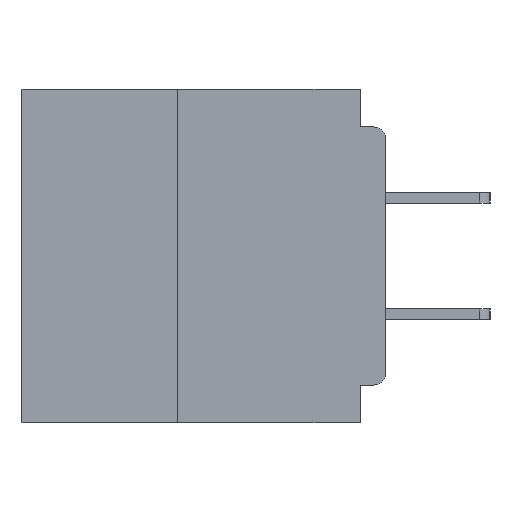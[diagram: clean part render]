
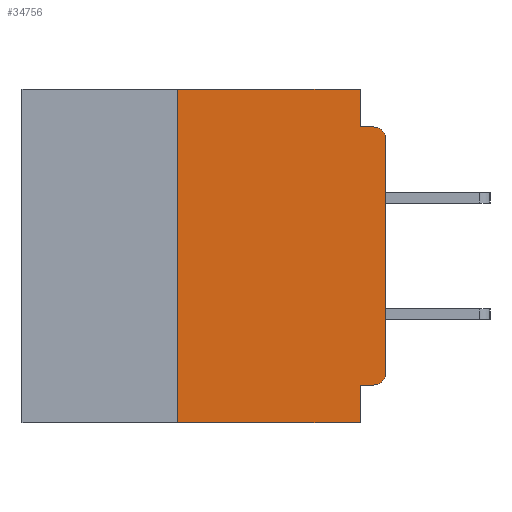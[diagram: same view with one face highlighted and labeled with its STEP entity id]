
A CAD part, left-side view. The second image highlights one B-rep face of the part: STEP entity #34756.
In plain terms, the highlighted planar face has unit normal (-1, 0, 0).
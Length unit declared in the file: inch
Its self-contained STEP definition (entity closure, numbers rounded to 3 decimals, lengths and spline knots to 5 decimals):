
#639 = LINE ( 'NONE', #32793, #15020 ) ;
#721 = ORIENTED_EDGE ( 'NONE', *, *, #3577, .T. ) ;
#1057 = ORIENTED_EDGE ( 'NONE', *, *, #13019, .F. ) ;
#1140 = ORIENTED_EDGE ( 'NONE', *, *, #12004, .T. ) ;
#1785 = VECTOR ( 'NONE', #26049, 39.37008 ) ;
#1883 = DIRECTION ( 'NONE',  ( 0., 0., -1. ) ) ;
#1894 = VERTEX_POINT ( 'NONE', #34865 ) ;
#2297 = DIRECTION ( 'NONE',  ( 0., 0., -1. ) ) ;
#2984 = CARTESIAN_POINT ( 'NONE',  ( 0., 0.031, -0.4 ) ) ;
#3577 = EDGE_CURVE ( 'NONE', #4861, #11537, #23771, .T. ) ;
#4065 = DIRECTION ( 'NONE',  ( 0., 0., -1. ) ) ;
#4103 = CARTESIAN_POINT ( 'NONE',  ( 0., 0.437, 0. ) ) ;
#4345 = EDGE_CURVE ( 'NONE', #21236, #17691, #6272, .T. ) ;
#4846 = ORIENTED_EDGE ( 'NONE', *, *, #19035, .F. ) ;
#4861 = VERTEX_POINT ( 'NONE', #14574 ) ;
#5144 = CARTESIAN_POINT ( 'NONE',  ( 0., 0.015, -0.045 ) ) ;
#5278 = FACE_OUTER_BOUND ( 'NONE', #33180, .T. ) ;
#5854 = AXIS2_PLACEMENT_3D ( 'NONE', #17732, #25345, #12584 ) ;
#6272 = CIRCLE ( 'NONE', #5854, 0.015 ) ;
#7004 = DIRECTION ( 'NONE',  ( 0., 0., -1. ) ) ;
#7488 = VECTOR ( 'NONE', #15208, 39.37008 ) ;
#8127 = LINE ( 'NONE', #34893, #23379 ) ;
#8141 = LINE ( 'NONE', #15370, #22509 ) ;
#9050 = ORIENTED_EDGE ( 'NONE', *, *, #25413, .F. ) ;
#9658 = CARTESIAN_POINT ( 'NONE',  ( 0., 0.031, -0.4 ) ) ;
#10877 = CARTESIAN_POINT ( 'NONE',  ( 0., 0., -0.06 ) ) ;
#11125 = AXIS2_PLACEMENT_3D ( 'NONE', #4103, #24119, #7004 ) ;
#11231 = EDGE_CURVE ( 'NONE', #4861, #1894, #639, .T. ) ;
#11537 = VERTEX_POINT ( 'NONE', #2984 ) ;
#11677 = ORIENTED_EDGE ( 'NONE', *, *, #16388, .T. ) ;
#12004 = EDGE_CURVE ( 'NONE', #18556, #16667, #25202, .T. ) ;
#12299 = CARTESIAN_POINT ( 'NONE',  ( 0., 0., 0. ) ) ;
#12584 = DIRECTION ( 'NONE',  ( 0., 0., -1. ) ) ;
#13019 = EDGE_CURVE ( 'NONE', #1894, #34013, #8127, .T. ) ;
#13176 = EDGE_CURVE ( 'NONE', #34013, #35790, #24674, .T. ) ;
#14282 = CARTESIAN_POINT ( 'NONE',  ( 0., 0., -0.355 ) ) ;
#14574 = CARTESIAN_POINT ( 'NONE',  ( 0., 0.25, -0.4 ) ) ;
#14696 = CARTESIAN_POINT ( 'NONE',  ( 0., 0.031, -0.045 ) ) ;
#15020 = VECTOR ( 'NONE', #35562, 39.37008 ) ;
#15208 = DIRECTION ( 'NONE',  ( 0., 0., 1. ) ) ;
#15370 = CARTESIAN_POINT ( 'NONE',  ( 0., 0., -0.045 ) ) ;
#15757 = ORIENTED_EDGE ( 'NONE', *, *, #31018, .F. ) ;
#15964 = VECTOR ( 'NONE', #4065, 39.37008 ) ;
#16388 = EDGE_CURVE ( 'NONE', #17691, #18556, #21843, .T. ) ;
#16667 = VERTEX_POINT ( 'NONE', #5144 ) ;
#17691 = VERTEX_POINT ( 'NONE', #24353 ) ;
#17732 = CARTESIAN_POINT ( 'NONE',  ( 0., 0.015, -0.34 ) ) ;
#18034 = VECTOR ( 'NONE', #1883, 39.37008 ) ;
#18426 = PLANE ( 'NONE',  #11125 ) ;
#18556 = VERTEX_POINT ( 'NONE', #10877 ) ;
#19035 = EDGE_CURVE ( 'NONE', #35790, #16667, #8141, .T. ) ;
#19127 = CARTESIAN_POINT ( 'NONE',  ( 0., 0.031, 0. ) ) ;
#19538 = DIRECTION ( 'NONE',  ( -1., 0., 0. ) ) ;
#20103 = ORIENTED_EDGE ( 'NONE', *, *, #4345, .T. ) ;
#20593 = CARTESIAN_POINT ( 'NONE',  ( 0., 0.031, 0. ) ) ;
#20868 = DIRECTION ( 'NONE',  ( 0., -1., 0. ) ) ;
#21149 = DIRECTION ( 'NONE',  ( 0., -1., 0. ) ) ;
#21236 = VERTEX_POINT ( 'NONE', #31223 ) ;
#21843 = LINE ( 'NONE', #12299, #7488 ) ;
#22329 = VECTOR ( 'NONE', #34121, 39.37008 ) ;
#22509 = VECTOR ( 'NONE', #21149, 39.37008 ) ;
#23379 = VECTOR ( 'NONE', #20868, 39.37008 ) ;
#23548 = LINE ( 'NONE', #9658, #15964 ) ;
#23771 = LINE ( 'NONE', #34441, #1785 ) ;
#24119 = DIRECTION ( 'NONE',  ( 1., 0., 0. ) ) ;
#24163 = VERTEX_POINT ( 'NONE', #29980 ) ;
#24353 = CARTESIAN_POINT ( 'NONE',  ( 0., 0., -0.34 ) ) ;
#24674 = LINE ( 'NONE', #19127, #18034 ) ;
#25202 = CIRCLE ( 'NONE', #29924, 0.015 ) ;
#25345 = DIRECTION ( 'NONE',  ( -1., 0., 0. ) ) ;
#25413 = EDGE_CURVE ( 'NONE', #21236, #24163, #29815, .T. ) ;
#26049 = DIRECTION ( 'NONE',  ( 0., -1., 0. ) ) ;
#26794 = ORIENTED_EDGE ( 'NONE', *, *, #13176, .F. ) ;
#28056 = ORIENTED_EDGE ( 'NONE', *, *, #11231, .F. ) ;
#29815 = LINE ( 'NONE', #14282, #22329 ) ;
#29924 = AXIS2_PLACEMENT_3D ( 'NONE', #36354, #19538, #2297 ) ;
#29980 = CARTESIAN_POINT ( 'NONE',  ( 0., 0.031, -0.355 ) ) ;
#31018 = EDGE_CURVE ( 'NONE', #24163, #11537, #23548, .T. ) ;
#31223 = CARTESIAN_POINT ( 'NONE',  ( 0., 0.015, -0.355 ) ) ;
#32793 = CARTESIAN_POINT ( 'NONE',  ( 0., 0.25, -0.4 ) ) ;
#33180 = EDGE_LOOP ( 'NONE', ( #11677, #1140, #4846, #26794, #1057, #28056, #721, #15757, #9050, #20103 ) ) ;
#34013 = VERTEX_POINT ( 'NONE', #20593 ) ;
#34121 = DIRECTION ( 'NONE',  ( 0., 1., 0. ) ) ;
#34441 = CARTESIAN_POINT ( 'NONE',  ( 0., 0.437, -0.4 ) ) ;
#34756 = ADVANCED_FACE ( 'NONE', ( #5278 ), #18426, .F. ) ;
#34865 = CARTESIAN_POINT ( 'NONE',  ( 0., 0.25, 0. ) ) ;
#34893 = CARTESIAN_POINT ( 'NONE',  ( 0., 0.437, 0. ) ) ;
#35562 = DIRECTION ( 'NONE',  ( 0., 0., 1. ) ) ;
#35790 = VERTEX_POINT ( 'NONE', #14696 ) ;
#36354 = CARTESIAN_POINT ( 'NONE',  ( 0., 0.015, -0.06 ) ) ;
